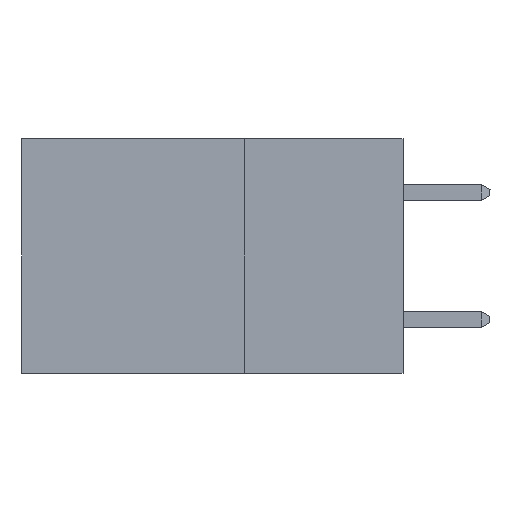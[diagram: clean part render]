
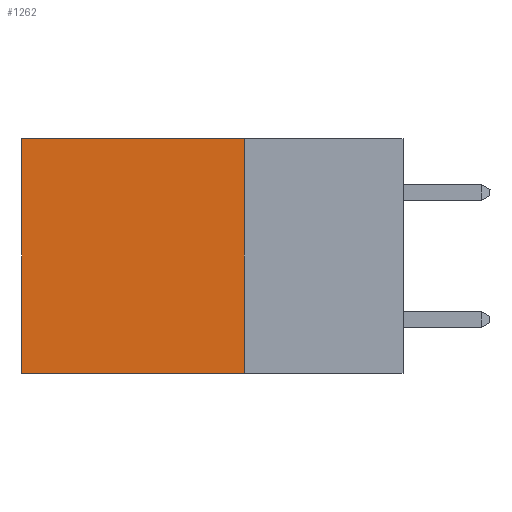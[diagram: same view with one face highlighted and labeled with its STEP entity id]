
A CAD part, left-side view. The second image highlights one B-rep face of the part: STEP entity #1262.
In plain terms, the highlighted planar face has unit normal (-1, 0, 0).
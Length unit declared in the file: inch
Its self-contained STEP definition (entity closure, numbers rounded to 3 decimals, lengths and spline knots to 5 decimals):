
#83 = CARTESIAN_POINT ( 'NONE',  ( 0.2875, 0.25, 0. ) ) ;
#419 = EDGE_CURVE ( 'NONE', #14686, #2168, #5267, .T. ) ;
#457 = LINE ( 'NONE', #13421, #10437 ) ;
#967 = CARTESIAN_POINT ( 'NONE',  ( 0.2875, 0.6, 0. ) ) ;
#1080 = AXIS2_PLACEMENT_3D ( 'NONE', #5223, #11251, #13554 ) ;
#1262 = ADVANCED_FACE ( 'NONE', ( #10064 ), #14642, .F. ) ;
#1849 = CARTESIAN_POINT ( 'NONE',  ( 0.2875, 0.25, 0. ) ) ;
#2168 = VERTEX_POINT ( 'NONE', #967 ) ;
#2848 = ORIENTED_EDGE ( 'NONE', *, *, #419, .T. ) ;
#3690 = DIRECTION ( 'NONE',  ( 0., 0., -1. ) ) ;
#4163 = VECTOR ( 'NONE', #3690, 39.37008 ) ;
#4693 = CARTESIAN_POINT ( 'NONE',  ( 0.2875, 0.6, -0.37 ) ) ;
#4905 = LINE ( 'NONE', #83, #4163 ) ;
#5015 = DIRECTION ( 'NONE',  ( 0., 1., 0. ) ) ;
#5223 = CARTESIAN_POINT ( 'NONE',  ( 0.2875, 0.25, 0. ) ) ;
#5267 = LINE ( 'NONE', #12512, #8057 ) ;
#5460 = VECTOR ( 'NONE', #5015, 39.37008 ) ;
#6332 = ORIENTED_EDGE ( 'NONE', *, *, #9817, .T. ) ;
#6615 = EDGE_LOOP ( 'NONE', ( #6332, #14341, #14840, #2848 ) ) ;
#7723 = DIRECTION ( 'NONE',  ( 0., 1., 0. ) ) ;
#8057 = VECTOR ( 'NONE', #7723, 39.37008 ) ;
#8769 = VERTEX_POINT ( 'NONE', #13882 ) ;
#9173 = EDGE_CURVE ( 'NONE', #8769, #10647, #13037, .T. ) ;
#9817 = EDGE_CURVE ( 'NONE', #2168, #10647, #457, .T. ) ;
#10064 = FACE_OUTER_BOUND ( 'NONE', #6615, .T. ) ;
#10437 = VECTOR ( 'NONE', #14569, 39.37008 ) ;
#10647 = VERTEX_POINT ( 'NONE', #4693 ) ;
#11251 = DIRECTION ( 'NONE',  ( 1., 0., 0. ) ) ;
#12087 = CARTESIAN_POINT ( 'NONE',  ( 0.2875, 0.25, -0.37 ) ) ;
#12512 = CARTESIAN_POINT ( 'NONE',  ( 0.2875, 0.25, 0. ) ) ;
#13037 = LINE ( 'NONE', #12087, #5460 ) ;
#13421 = CARTESIAN_POINT ( 'NONE',  ( 0.2875, 0.6, 0. ) ) ;
#13554 = DIRECTION ( 'NONE',  ( 0., 0., -1. ) ) ;
#13882 = CARTESIAN_POINT ( 'NONE',  ( 0.2875, 0.25, -0.37 ) ) ;
#14341 = ORIENTED_EDGE ( 'NONE', *, *, #9173, .F. ) ;
#14569 = DIRECTION ( 'NONE',  ( 0., 0., -1. ) ) ;
#14642 = PLANE ( 'NONE',  #1080 ) ;
#14686 = VERTEX_POINT ( 'NONE', #1849 ) ;
#14840 = ORIENTED_EDGE ( 'NONE', *, *, #14975, .F. ) ;
#14975 = EDGE_CURVE ( 'NONE', #14686, #8769, #4905, .T. ) ;
